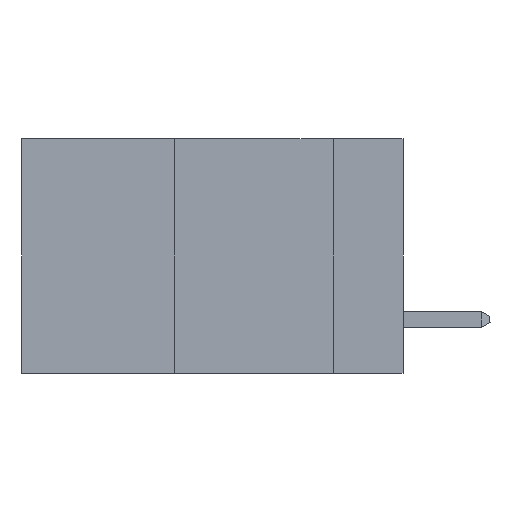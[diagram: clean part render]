
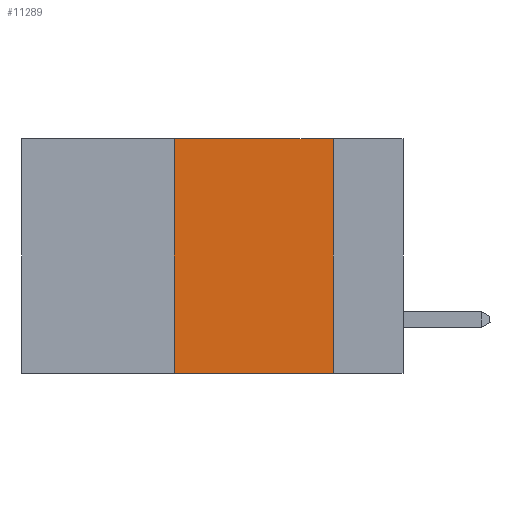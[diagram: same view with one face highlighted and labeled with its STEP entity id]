
A CAD part, left-side view. The second image highlights one B-rep face of the part: STEP entity #11289.
In plain terms, the highlighted planar face has unit normal (-1, 0, 0).
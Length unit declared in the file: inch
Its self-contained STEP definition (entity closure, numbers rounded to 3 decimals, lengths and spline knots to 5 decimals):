
#51 = EDGE_CURVE ( 'NONE', #14110, #7308, #7373, .T. ) ;
#472 = CARTESIAN_POINT ( 'NONE',  ( 0., 0.36, 0. ) ) ;
#990 = CARTESIAN_POINT ( 'NONE',  ( 0., 0.36, -0.37 ) ) ;
#1398 = CARTESIAN_POINT ( 'NONE',  ( 0., 0.11, 0. ) ) ;
#1585 = EDGE_CURVE ( 'NONE', #19452, #6331, #19309, .T. ) ;
#1631 = DIRECTION ( 'NONE',  ( 0., 0., -1. ) ) ;
#2625 = VECTOR ( 'NONE', #20882, 39.37008 ) ;
#4923 = CARTESIAN_POINT ( 'NONE',  ( 0., 0.6, -0.37 ) ) ;
#5283 = DIRECTION ( 'NONE',  ( 0., 0., -1. ) ) ;
#5645 = CARTESIAN_POINT ( 'NONE',  ( 0., 0.11, -0.37 ) ) ;
#6331 = VERTEX_POINT ( 'NONE', #5645 ) ;
#6943 = PLANE ( 'NONE',  #8863 ) ;
#7308 = VERTEX_POINT ( 'NONE', #1398 ) ;
#7373 = LINE ( 'NONE', #8422, #2625 ) ;
#7876 = LINE ( 'NONE', #12077, #19591 ) ;
#8321 = DIRECTION ( 'NONE',  ( 0., 0., 1. ) ) ;
#8422 = CARTESIAN_POINT ( 'NONE',  ( 0., 0.6, 0. ) ) ;
#8863 = AXIS2_PLACEMENT_3D ( 'NONE', #14208, #15955, #5283 ) ;
#10286 = CARTESIAN_POINT ( 'NONE',  ( 0., 0.11, 0. ) ) ;
#10698 = EDGE_CURVE ( 'NONE', #7308, #6331, #10828, .T. ) ;
#10828 = LINE ( 'NONE', #10286, #18267 ) ;
#11289 = ADVANCED_FACE ( 'NONE', ( #18549 ), #6943, .F. ) ;
#11560 = EDGE_LOOP ( 'NONE', ( #22088, #16299, #22734, #15054 ) ) ;
#12077 = CARTESIAN_POINT ( 'NONE',  ( 0., 0.36, 0. ) ) ;
#14110 = VERTEX_POINT ( 'NONE', #472 ) ;
#14208 = CARTESIAN_POINT ( 'NONE',  ( 0., 0.6, 0. ) ) ;
#15054 = ORIENTED_EDGE ( 'NONE', *, *, #1585, .T. ) ;
#15441 = DIRECTION ( 'NONE',  ( 0., -1., 0. ) ) ;
#15955 = DIRECTION ( 'NONE',  ( 1., 0., 0. ) ) ;
#16299 = ORIENTED_EDGE ( 'NONE', *, *, #51, .F. ) ;
#17052 = VECTOR ( 'NONE', #15441, 39.37008 ) ;
#17795 = EDGE_CURVE ( 'NONE', #19452, #14110, #7876, .T. ) ;
#18267 = VECTOR ( 'NONE', #1631, 39.37008 ) ;
#18549 = FACE_OUTER_BOUND ( 'NONE', #11560, .T. ) ;
#19309 = LINE ( 'NONE', #4923, #17052 ) ;
#19452 = VERTEX_POINT ( 'NONE', #990 ) ;
#19591 = VECTOR ( 'NONE', #8321, 39.37008 ) ;
#20882 = DIRECTION ( 'NONE',  ( 0., -1., 0. ) ) ;
#22088 = ORIENTED_EDGE ( 'NONE', *, *, #10698, .F. ) ;
#22734 = ORIENTED_EDGE ( 'NONE', *, *, #17795, .F. ) ;
